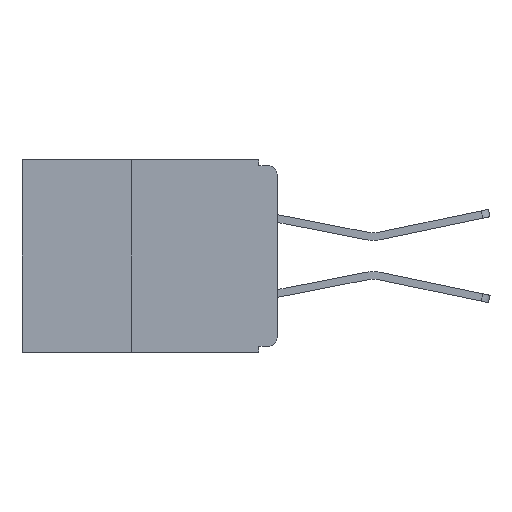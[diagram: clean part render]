
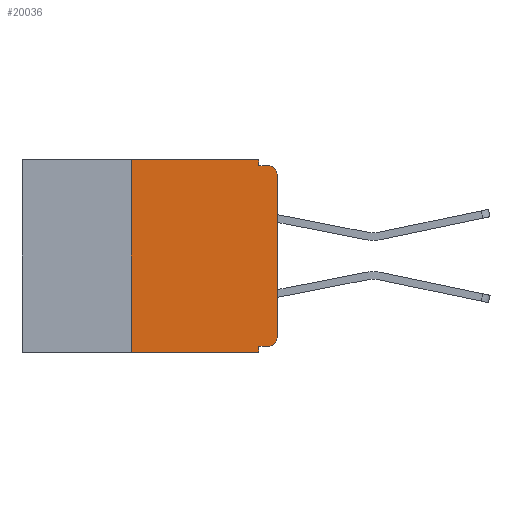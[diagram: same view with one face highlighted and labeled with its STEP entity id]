
A CAD part, left-side view. The second image highlights one B-rep face of the part: STEP entity #20036.
In plain terms, the highlighted planar face has unit normal (-1, 0, 0).
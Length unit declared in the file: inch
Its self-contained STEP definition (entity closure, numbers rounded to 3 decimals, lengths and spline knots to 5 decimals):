
#269 = EDGE_CURVE ( 'NONE', #3734, #13450, #1121, .T. ) ;
#404 = VERTEX_POINT ( 'NONE', #16244 ) ;
#682 = VECTOR ( 'NONE', #4770, 39.37008 ) ;
#924 = AXIS2_PLACEMENT_3D ( 'NONE', #14699, #33235, #17426 ) ;
#982 = DIRECTION ( 'NONE',  ( 0., 0., -1. ) ) ;
#1121 = LINE ( 'NONE', #8088, #21278 ) ;
#1163 = ORIENTED_EDGE ( 'NONE', *, *, #15291, .F. ) ;
#1738 = VERTEX_POINT ( 'NONE', #11089 ) ;
#1765 = DIRECTION ( 'NONE',  ( 0., 1., 0. ) ) ;
#1985 = CARTESIAN_POINT ( 'NONE',  ( 0., 0.031, -0.33 ) ) ;
#2395 = DIRECTION ( 'NONE',  ( 0., 0., -1. ) ) ;
#3734 = VERTEX_POINT ( 'NONE', #25867 ) ;
#3943 = CIRCLE ( 'NONE', #924, 0.015 ) ;
#4173 = VECTOR ( 'NONE', #2395, 39.37008 ) ;
#4738 = PLANE ( 'NONE',  #28677 ) ;
#4770 = DIRECTION ( 'NONE',  ( 0., 0., -1. ) ) ;
#4988 = CARTESIAN_POINT ( 'NONE',  ( 0., 0.25, -0.33 ) ) ;
#5413 = ORIENTED_EDGE ( 'NONE', *, *, #20427, .F. ) ;
#5872 = ORIENTED_EDGE ( 'NONE', *, *, #7224, .F. ) ;
#6430 = DIRECTION ( 'NONE',  ( 0., -1., 0. ) ) ;
#6685 = EDGE_CURVE ( 'NONE', #6865, #3734, #12369, .T. ) ;
#6865 = VERTEX_POINT ( 'NONE', #16970 ) ;
#6942 = LINE ( 'NONE', #10851, #27653 ) ;
#7224 = EDGE_CURVE ( 'NONE', #19607, #404, #8074, .T. ) ;
#7554 = DIRECTION ( 'NONE',  ( 1., 0., 0. ) ) ;
#8074 = LINE ( 'NONE', #1985, #682 ) ;
#8088 = CARTESIAN_POINT ( 'NONE',  ( 0., 0., -0.01 ) ) ;
#8352 = CARTESIAN_POINT ( 'NONE',  ( 0., 0.437, -0.33 ) ) ;
#8742 = DIRECTION ( 'NONE',  ( 0., 0., 1. ) ) ;
#8844 = FACE_OUTER_BOUND ( 'NONE', #19913, .T. ) ;
#9224 = DIRECTION ( 'NONE',  ( 0., -1., 0. ) ) ;
#9851 = EDGE_CURVE ( 'NONE', #1738, #13450, #3943, .T. ) ;
#10851 = CARTESIAN_POINT ( 'NONE',  ( 0., 0., 0. ) ) ;
#11089 = CARTESIAN_POINT ( 'NONE',  ( 0., 0., -0.025 ) ) ;
#11125 = CIRCLE ( 'NONE', #21604, 0.015 ) ;
#12369 = LINE ( 'NONE', #21562, #4173 ) ;
#12764 = VERTEX_POINT ( 'NONE', #33142 ) ;
#13450 = VERTEX_POINT ( 'NONE', #30577 ) ;
#13636 = DIRECTION ( 'NONE',  ( 0., 0., 1. ) ) ;
#14006 = VECTOR ( 'NONE', #1765, 39.37008 ) ;
#14485 = CARTESIAN_POINT ( 'NONE',  ( 0., 0.015, -0.32 ) ) ;
#14566 = EDGE_CURVE ( 'NONE', #24781, #404, #16203, .T. ) ;
#14628 = CARTESIAN_POINT ( 'NONE',  ( 0., 0.437, 0. ) ) ;
#14699 = CARTESIAN_POINT ( 'NONE',  ( 0., 0.015, -0.025 ) ) ;
#15291 = EDGE_CURVE ( 'NONE', #19079, #19607, #21205, .T. ) ;
#15534 = CARTESIAN_POINT ( 'NONE',  ( 0., 0., -0.32 ) ) ;
#15751 = ORIENTED_EDGE ( 'NONE', *, *, #29157, .T. ) ;
#16203 = LINE ( 'NONE', #8352, #29485 ) ;
#16244 = CARTESIAN_POINT ( 'NONE',  ( 0., 0.031, -0.33 ) ) ;
#16585 = LINE ( 'NONE', #27590, #29852 ) ;
#16970 = CARTESIAN_POINT ( 'NONE',  ( 0., 0.031, 0. ) ) ;
#17426 = DIRECTION ( 'NONE',  ( 0., 0., -1. ) ) ;
#17471 = DIRECTION ( 'NONE',  ( -1., 0., 0. ) ) ;
#19079 = VERTEX_POINT ( 'NONE', #14485 ) ;
#19607 = VERTEX_POINT ( 'NONE', #27401 ) ;
#19913 = EDGE_LOOP ( 'NONE', ( #15751, #30288, #24937, #24534, #5413, #31131, #33601, #5872, #1163, #25465 ) ) ;
#20036 = ADVANCED_FACE ( 'NONE', ( #8844 ), #4738, .F. ) ;
#20427 = EDGE_CURVE ( 'NONE', #21311, #6865, #24028, .T. ) ;
#21205 = LINE ( 'NONE', #15534, #14006 ) ;
#21278 = VECTOR ( 'NONE', #6430, 39.37008 ) ;
#21311 = VERTEX_POINT ( 'NONE', #24629 ) ;
#21562 = CARTESIAN_POINT ( 'NONE',  ( 0., 0.031, 0. ) ) ;
#21604 = AXIS2_PLACEMENT_3D ( 'NONE', #33290, #17471, #982 ) ;
#23221 = VECTOR ( 'NONE', #9224, 39.37008 ) ;
#23778 = CARTESIAN_POINT ( 'NONE',  ( 0., 0.437, 0. ) ) ;
#24028 = LINE ( 'NONE', #14628, #23221 ) ;
#24534 = ORIENTED_EDGE ( 'NONE', *, *, #6685, .F. ) ;
#24629 = CARTESIAN_POINT ( 'NONE',  ( 0., 0.25, 0. ) ) ;
#24781 = VERTEX_POINT ( 'NONE', #4988 ) ;
#24937 = ORIENTED_EDGE ( 'NONE', *, *, #269, .F. ) ;
#25465 = ORIENTED_EDGE ( 'NONE', *, *, #30366, .T. ) ;
#25867 = CARTESIAN_POINT ( 'NONE',  ( 0., 0.031, -0.01 ) ) ;
#26447 = DIRECTION ( 'NONE',  ( 0., 0., -1. ) ) ;
#27195 = DIRECTION ( 'NONE',  ( 0., -1., 0. ) ) ;
#27401 = CARTESIAN_POINT ( 'NONE',  ( 0., 0.031, -0.32 ) ) ;
#27590 = CARTESIAN_POINT ( 'NONE',  ( 0., 0.25, -0.33 ) ) ;
#27653 = VECTOR ( 'NONE', #13636, 39.37008 ) ;
#28677 = AXIS2_PLACEMENT_3D ( 'NONE', #23778, #7554, #26447 ) ;
#29157 = EDGE_CURVE ( 'NONE', #12764, #1738, #6942, .T. ) ;
#29485 = VECTOR ( 'NONE', #27195, 39.37008 ) ;
#29852 = VECTOR ( 'NONE', #8742, 39.37008 ) ;
#30288 = ORIENTED_EDGE ( 'NONE', *, *, #9851, .T. ) ;
#30366 = EDGE_CURVE ( 'NONE', #19079, #12764, #11125, .T. ) ;
#30577 = CARTESIAN_POINT ( 'NONE',  ( 0., 0.015, -0.01 ) ) ;
#31131 = ORIENTED_EDGE ( 'NONE', *, *, #32577, .F. ) ;
#32577 = EDGE_CURVE ( 'NONE', #24781, #21311, #16585, .T. ) ;
#33142 = CARTESIAN_POINT ( 'NONE',  ( 0., 0., -0.305 ) ) ;
#33235 = DIRECTION ( 'NONE',  ( -1., 0., 0. ) ) ;
#33290 = CARTESIAN_POINT ( 'NONE',  ( 0., 0.015, -0.305 ) ) ;
#33601 = ORIENTED_EDGE ( 'NONE', *, *, #14566, .T. ) ;
